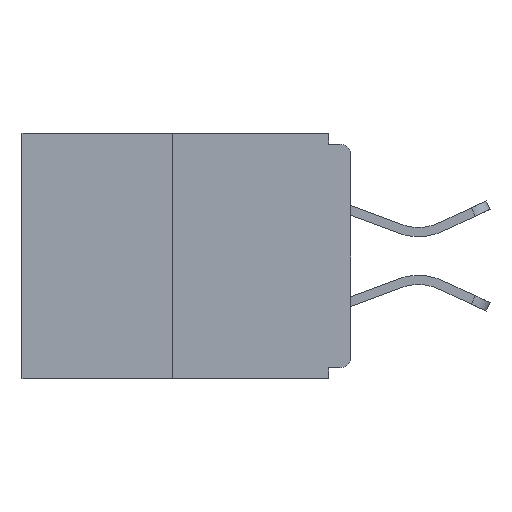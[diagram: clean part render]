
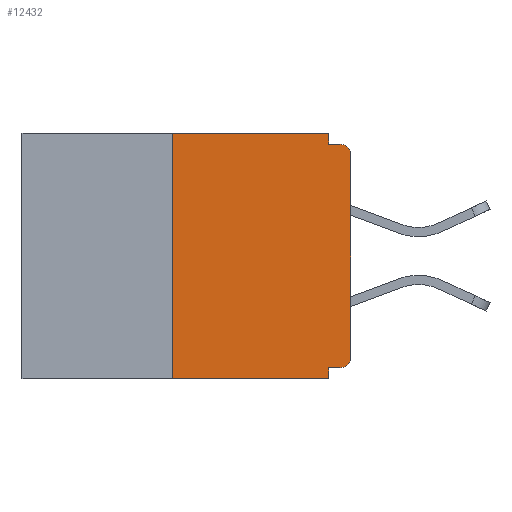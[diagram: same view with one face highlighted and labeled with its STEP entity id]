
A CAD part, left-side view. The second image highlights one B-rep face of the part: STEP entity #12432.
In plain terms, the highlighted planar face has unit normal (-1, 0, 0).
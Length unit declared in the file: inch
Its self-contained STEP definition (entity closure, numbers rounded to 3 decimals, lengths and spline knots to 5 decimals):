
#320 = VERTEX_POINT ( 'NONE', #3369 ) ;
#405 = DIRECTION ( 'NONE',  ( 0., -1., 0. ) ) ;
#645 = DIRECTION ( 'NONE',  ( 0., 0., -1. ) ) ;
#715 = EDGE_CURVE ( 'NONE', #22608, #17469, #26927, .T. ) ;
#1125 = EDGE_CURVE ( 'NONE', #17469, #28558, #24467, .T. ) ;
#1236 = ORIENTED_EDGE ( 'NONE', *, *, #27271, .F. ) ;
#1456 = LINE ( 'NONE', #15636, #24335 ) ;
#3156 = CIRCLE ( 'NONE', #5374, 0.015 ) ;
#3234 = ORIENTED_EDGE ( 'NONE', *, *, #25058, .F. ) ;
#3369 = CARTESIAN_POINT ( 'NONE',  ( 0., 0., -0.03 ) ) ;
#3471 = EDGE_CURVE ( 'NONE', #25056, #6559, #3156, .T. ) ;
#3490 = CARTESIAN_POINT ( 'NONE',  ( 0., 0.031, 0. ) ) ;
#4322 = CARTESIAN_POINT ( 'NONE',  ( 0., 0., -0.328 ) ) ;
#4376 = VERTEX_POINT ( 'NONE', #21404 ) ;
#4894 = CARTESIAN_POINT ( 'NONE',  ( 0., 0.031, -0.328 ) ) ;
#5131 = ORIENTED_EDGE ( 'NONE', *, *, #715, .F. ) ;
#5374 = AXIS2_PLACEMENT_3D ( 'NONE', #19927, #22085, #17809 ) ;
#5521 = CARTESIAN_POINT ( 'NONE',  ( 0., 0.031, -0.343 ) ) ;
#5524 = LINE ( 'NONE', #20011, #22229 ) ;
#5772 = AXIS2_PLACEMENT_3D ( 'NONE', #10310, #12535, #14768 ) ;
#5837 = CARTESIAN_POINT ( 'NONE',  ( 0., 0.031, -0.015 ) ) ;
#6151 = EDGE_CURVE ( 'NONE', #6559, #320, #11330, .T. ) ;
#6559 = VERTEX_POINT ( 'NONE', #20660 ) ;
#6804 = LINE ( 'NONE', #22371, #19999 ) ;
#8015 = DIRECTION ( 'NONE',  ( 0., 0., -1. ) ) ;
#8715 = ORIENTED_EDGE ( 'NONE', *, *, #1125, .F. ) ;
#8783 = ORIENTED_EDGE ( 'NONE', *, *, #23031, .T. ) ;
#9260 = ORIENTED_EDGE ( 'NONE', *, *, #3471, .T. ) ;
#9305 = DIRECTION ( 'NONE',  ( 1., 0., 0. ) ) ;
#10135 = DIRECTION ( 'NONE',  ( 0., 0., 1. ) ) ;
#10302 = CARTESIAN_POINT ( 'NONE',  ( 0., 0.031, 0. ) ) ;
#10310 = CARTESIAN_POINT ( 'NONE',  ( 0., 0.015, -0.03 ) ) ;
#11330 = LINE ( 'NONE', #19415, #21780 ) ;
#11471 = CARTESIAN_POINT ( 'NONE',  ( 0., 0.46, 0. ) ) ;
#12432 = ADVANCED_FACE ( 'NONE', ( #12539 ), #18163, .F. ) ;
#12535 = DIRECTION ( 'NONE',  ( -1., 0., 0. ) ) ;
#12539 = FACE_OUTER_BOUND ( 'NONE', #28422, .T. ) ;
#13223 = DIRECTION ( 'NONE',  ( 0., -1., 0. ) ) ;
#13381 = CARTESIAN_POINT ( 'NONE',  ( 0., 0.25, 0. ) ) ;
#13684 = CARTESIAN_POINT ( 'NONE',  ( 0., 0.015, -0.328 ) ) ;
#13854 = CARTESIAN_POINT ( 'NONE',  ( 0., 0.46, 0. ) ) ;
#13921 = ORIENTED_EDGE ( 'NONE', *, *, #21216, .F. ) ;
#14211 = CARTESIAN_POINT ( 'NONE',  ( 0., 0.25, 0. ) ) ;
#14256 = VECTOR ( 'NONE', #21989, 39.37008 ) ;
#14266 = AXIS2_PLACEMENT_3D ( 'NONE', #13854, #9305, #645 ) ;
#14768 = DIRECTION ( 'NONE',  ( 0., 0., -1. ) ) ;
#14957 = LINE ( 'NONE', #4322, #14256 ) ;
#15099 = DIRECTION ( 'NONE',  ( 0., 0., 1. ) ) ;
#15193 = EDGE_CURVE ( 'NONE', #320, #4376, #23530, .T. ) ;
#15636 = CARTESIAN_POINT ( 'NONE',  ( 0., 0., -0.015 ) ) ;
#17136 = VECTOR ( 'NONE', #8015, 39.37008 ) ;
#17469 = VERTEX_POINT ( 'NONE', #13381 ) ;
#17809 = DIRECTION ( 'NONE',  ( 0., 0., -1. ) ) ;
#18163 = PLANE ( 'NONE',  #14266 ) ;
#18275 = ORIENTED_EDGE ( 'NONE', *, *, #26690, .F. ) ;
#18540 = LINE ( 'NONE', #3490, #17136 ) ;
#19282 = VECTOR ( 'NONE', #405, 39.37008 ) ;
#19415 = CARTESIAN_POINT ( 'NONE',  ( 0., 0., 0. ) ) ;
#19927 = CARTESIAN_POINT ( 'NONE',  ( 0., 0.015, -0.313 ) ) ;
#19999 = VECTOR ( 'NONE', #24569, 39.37008 ) ;
#20011 = CARTESIAN_POINT ( 'NONE',  ( 0., 0.031, -0.343 ) ) ;
#20660 = CARTESIAN_POINT ( 'NONE',  ( 0., 0., -0.313 ) ) ;
#21070 = VECTOR ( 'NONE', #10135, 39.37008 ) ;
#21216 = EDGE_CURVE ( 'NONE', #24443, #27901, #5524, .T. ) ;
#21404 = CARTESIAN_POINT ( 'NONE',  ( 0., 0.015, -0.015 ) ) ;
#21780 = VECTOR ( 'NONE', #15099, 39.37008 ) ;
#21989 = DIRECTION ( 'NONE',  ( 0., 1., 0. ) ) ;
#22085 = DIRECTION ( 'NONE',  ( -1., 0., 0. ) ) ;
#22229 = VECTOR ( 'NONE', #24757, 39.37008 ) ;
#22371 = CARTESIAN_POINT ( 'NONE',  ( 0., 0.46, -0.343 ) ) ;
#22456 = ORIENTED_EDGE ( 'NONE', *, *, #15193, .T. ) ;
#22608 = VERTEX_POINT ( 'NONE', #26803 ) ;
#23031 = EDGE_CURVE ( 'NONE', #22608, #27901, #6804, .T. ) ;
#23530 = CIRCLE ( 'NONE', #5772, 0.015 ) ;
#24335 = VECTOR ( 'NONE', #13223, 39.37008 ) ;
#24443 = VERTEX_POINT ( 'NONE', #4894 ) ;
#24467 = LINE ( 'NONE', #11471, #19282 ) ;
#24569 = DIRECTION ( 'NONE',  ( 0., -1., 0. ) ) ;
#24757 = DIRECTION ( 'NONE',  ( 0., 0., -1. ) ) ;
#25056 = VERTEX_POINT ( 'NONE', #13684 ) ;
#25058 = EDGE_CURVE ( 'NONE', #28558, #26974, #18540, .T. ) ;
#25545 = ORIENTED_EDGE ( 'NONE', *, *, #6151, .T. ) ;
#26690 = EDGE_CURVE ( 'NONE', #25056, #24443, #14957, .T. ) ;
#26803 = CARTESIAN_POINT ( 'NONE',  ( 0., 0.25, -0.343 ) ) ;
#26927 = LINE ( 'NONE', #14211, #21070 ) ;
#26974 = VERTEX_POINT ( 'NONE', #5837 ) ;
#27271 = EDGE_CURVE ( 'NONE', #26974, #4376, #1456, .T. ) ;
#27901 = VERTEX_POINT ( 'NONE', #5521 ) ;
#28422 = EDGE_LOOP ( 'NONE', ( #8715, #5131, #8783, #13921, #18275, #9260, #25545, #22456, #1236, #3234 ) ) ;
#28558 = VERTEX_POINT ( 'NONE', #10302 ) ;
